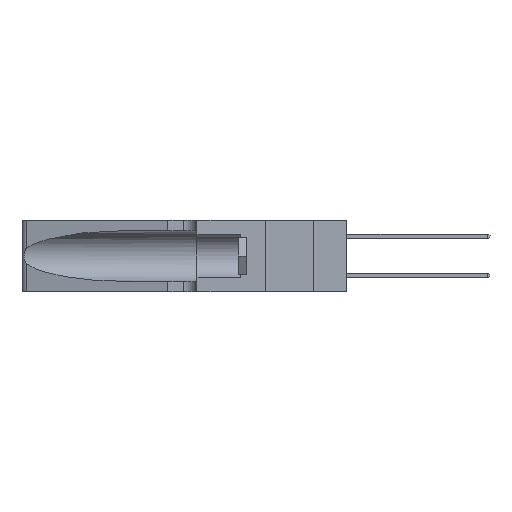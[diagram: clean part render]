
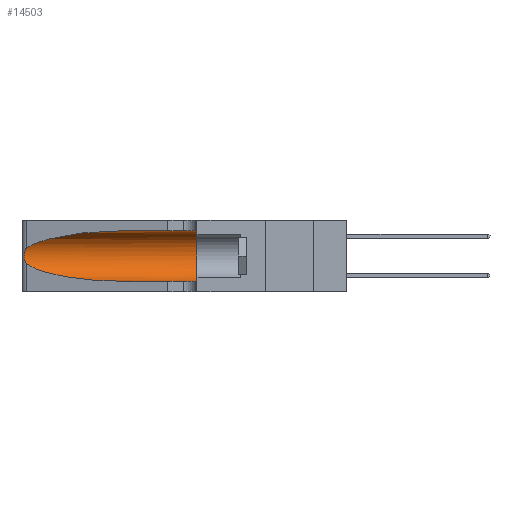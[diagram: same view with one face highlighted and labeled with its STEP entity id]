
A CAD part, left-side view. The second image highlights one B-rep face of the part: STEP entity #14503.
In plain terms, the highlighted cylindrical face has radius 3.308 mm (diameter 6.617 mm), a partial arc.
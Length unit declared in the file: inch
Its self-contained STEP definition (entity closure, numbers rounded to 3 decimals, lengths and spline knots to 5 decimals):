
#587 = EDGE_CURVE ( 'NONE', #1886, #10884, #25623, .T. ) ;
#595 = CARTESIAN_POINT ( 'NONE',  ( 0.26075, 1.23896, 0.19203 ) ) ;
#1101 = EDGE_CURVE ( 'NONE', #13649, #16654, #11084, .T. ) ;
#1199 = VECTOR ( 'NONE', #26943, 39.37008 ) ;
#1886 = VERTEX_POINT ( 'NONE', #23647 ) ;
#2947 = CARTESIAN_POINT ( 'NONE',  ( 0.25639, 1.23186, 0.15144 ) ) ;
#3329 = CARTESIAN_POINT ( 'NONE',  ( 0.1305, 0.35, 0.05475 ) ) ;
#4077 = EDGE_CURVE ( 'NONE', #21924, #1886, #8734, .T. ) ;
#4171 = CARTESIAN_POINT ( 'NONE',  ( 0.1305, 1.61858, 0.05475 ) ) ;
#5030 = CARTESIAN_POINT ( 'NONE',  ( 0.25787, 1.23484, 0.2124 ) ) ;
#5219 = CARTESIAN_POINT ( 'NONE',  ( 0.25555, 1.22993, 0.14849 ) ) ;
#5710 = CARTESIAN_POINT ( 'NONE',  ( 0.1305, 0.72297, 0.31525 ) ) ;
#6042 = CYLINDRICAL_SURFACE ( 'NONE', #16323, 0.13025 ) ;
#7202 = VERTEX_POINT ( 'NONE', #27152 ) ;
#7459 = FACE_OUTER_BOUND ( 'NONE', #9987, .T. ) ;
#7682 = CARTESIAN_POINT ( 'NONE',  ( 0.26017, 1.23833, 0.17102 ) ) ;
#8127 = ORIENTED_EDGE ( 'NONE', *, *, #11458, .F. ) ;
#8203 =( BOUNDED_CURVE ( )  B_SPLINE_CURVE ( 3, ( #5710, #8372, #15006, #28728 ),
 .UNSPECIFIED., .F., .F. ) 
 B_SPLINE_CURVE_WITH_KNOTS ( ( 4, 4 ),
 ( 1.5708, 2.84003 ),
 .UNSPECIFIED. ) 
 CURVE ( )  GEOMETRIC_REPRESENTATION_ITEM ( )  RATIONAL_B_SPLINE_CURVE ( ( 1., 0.87, 0.87, 1. ) ) 
 REPRESENTATION_ITEM ( '' )  );
#8372 = CARTESIAN_POINT ( 'NONE',  ( 0.18966, 0.96281, 0.31525 ) ) ;
#8566 = DIRECTION ( 'NONE',  ( 0., 0., 1. ) ) ;
#8734 =( BOUNDED_CURVE ( )  B_SPLINE_CURVE ( 3, ( #17150, #26221, #24136, #10314 ),
 .UNSPECIFIED., .F., .F. ) 
 B_SPLINE_CURVE_WITH_KNOTS ( ( 4, 4 ),
 ( 3.44316, 4.71239 ),
 .UNSPECIFIED. ) 
 CURVE ( )  GEOMETRIC_REPRESENTATION_ITEM ( )  RATIONAL_B_SPLINE_CURVE ( ( 1., 0.87, 0.87, 1. ) ) 
 REPRESENTATION_ITEM ( '' )  );
#8864 = CARTESIAN_POINT ( 'NONE',  ( 0.1305, 1.61858, 0.31525 ) ) ;
#9031 = EDGE_CURVE ( 'NONE', #13649, #7202, #8203, .T. ) ;
#9987 = EDGE_LOOP ( 'NONE', ( #28105, #20428, #23909, #17492, #8127, #10085 ) ) ;
#10085 = ORIENTED_EDGE ( 'NONE', *, *, #1101, .F. ) ;
#10314 = CARTESIAN_POINT ( 'NONE',  ( 0.1305, 0.72297, 0.05475 ) ) ;
#10560 = CARTESIAN_POINT ( 'NONE',  ( 0.1305, 0.35, 0.185 ) ) ;
#10656 = DIRECTION ( 'NONE',  ( 0., 1., 0. ) ) ;
#10884 = VERTEX_POINT ( 'NONE', #3329 ) ;
#11084 = LINE ( 'NONE', #8864, #1199 ) ;
#11458 = EDGE_CURVE ( 'NONE', #16654, #10884, #17827, .T. ) ;
#11637 = CARTESIAN_POINT ( 'NONE',  ( 0.1305, 0.72297, 0.31525 ) ) ;
#12138 = CARTESIAN_POINT ( 'NONE',  ( 0.25487, 1.22718, 0.14631 ) ) ;
#13002 = CARTESIAN_POINT ( 'NONE',  ( 0.1305, 1.61858, 0.185 ) ) ;
#13649 = VERTEX_POINT ( 'NONE', #11637 ) ;
#14363 = B_SPLINE_CURVE_WITH_KNOTS ( 'NONE', 3,
 ( #27346, #27926, #28024, #5030, #25372, #25462, #595, #16578, #7682, #18854, #18548, #2947, #5219, #12138 ),
 .UNSPECIFIED., .F., .F.,
 ( 4, 2, 2, 2, 2, 2, 4 ),
 ( 0., 0.00027, 0.00053, 0.00107, 0.0016, 0.00187, 0.00214 ),
 .UNSPECIFIED. ) ;
#14503 = ADVANCED_FACE ( 'NONE', ( #7459 ), #6042, .F. ) ;
#15006 = CARTESIAN_POINT ( 'NONE',  ( 0.2373, 1.15595, 0.28018 ) ) ;
#15336 = DIRECTION ( 'NONE',  ( 0., 0., -1. ) ) ;
#16323 = AXIS2_PLACEMENT_3D ( 'NONE', #13002, #26493, #15336 ) ;
#16578 = CARTESIAN_POINT ( 'NONE',  ( 0.26075, 1.23896, 0.178 ) ) ;
#16654 = VERTEX_POINT ( 'NONE', #26876 ) ;
#17150 = CARTESIAN_POINT ( 'NONE',  ( 0.25487, 1.22718, 0.14631 ) ) ;
#17492 = ORIENTED_EDGE ( 'NONE', *, *, #587, .T. ) ;
#17827 = CIRCLE ( 'NONE', #28576, 0.13025 ) ;
#18548 = CARTESIAN_POINT ( 'NONE',  ( 0.25789, 1.23486, 0.15765 ) ) ;
#18854 = CARTESIAN_POINT ( 'NONE',  ( 0.25856, 1.23593, 0.16098 ) ) ;
#20428 = ORIENTED_EDGE ( 'NONE', *, *, #21260, .T. ) ;
#21260 = EDGE_CURVE ( 'NONE', #7202, #21924, #14363, .T. ) ;
#21924 = VERTEX_POINT ( 'NONE', #27712 ) ;
#22786 = VECTOR ( 'NONE', #28863, 39.37008 ) ;
#23647 = CARTESIAN_POINT ( 'NONE',  ( 0.1305, 0.72297, 0.05475 ) ) ;
#23909 = ORIENTED_EDGE ( 'NONE', *, *, #4077, .T. ) ;
#24136 = CARTESIAN_POINT ( 'NONE',  ( 0.18966, 0.96281, 0.05475 ) ) ;
#25372 = CARTESIAN_POINT ( 'NONE',  ( 0.25854, 1.2359, 0.20912 ) ) ;
#25462 = CARTESIAN_POINT ( 'NONE',  ( 0.26018, 1.23835, 0.19895 ) ) ;
#25623 = LINE ( 'NONE', #4171, #22786 ) ;
#26221 = CARTESIAN_POINT ( 'NONE',  ( 0.2373, 1.15595, 0.08982 ) ) ;
#26493 = DIRECTION ( 'NONE',  ( 0., -1., 0. ) ) ;
#26876 = CARTESIAN_POINT ( 'NONE',  ( 0.1305, 0.35, 0.31525 ) ) ;
#26943 = DIRECTION ( 'NONE',  ( 0., -1., 0. ) ) ;
#27152 = CARTESIAN_POINT ( 'NONE',  ( 0.25487, 1.22718, 0.22369 ) ) ;
#27346 = CARTESIAN_POINT ( 'NONE',  ( 0.25487, 1.22718, 0.22369 ) ) ;
#27712 = CARTESIAN_POINT ( 'NONE',  ( 0.25487, 1.22718, 0.14631 ) ) ;
#27926 = CARTESIAN_POINT ( 'NONE',  ( 0.25555, 1.22994, 0.2215 ) ) ;
#28024 = CARTESIAN_POINT ( 'NONE',  ( 0.25639, 1.23184, 0.21858 ) ) ;
#28105 = ORIENTED_EDGE ( 'NONE', *, *, #9031, .T. ) ;
#28576 = AXIS2_PLACEMENT_3D ( 'NONE', #10560, #10656, #8566 ) ;
#28728 = CARTESIAN_POINT ( 'NONE',  ( 0.25487, 1.22718, 0.22369 ) ) ;
#28863 = DIRECTION ( 'NONE',  ( 0., -1., 0. ) ) ;
